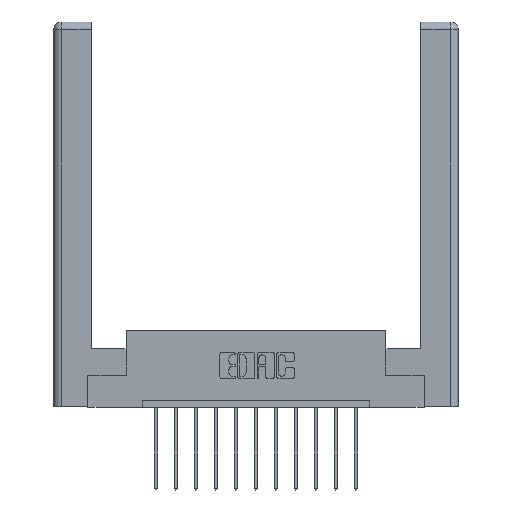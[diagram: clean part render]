
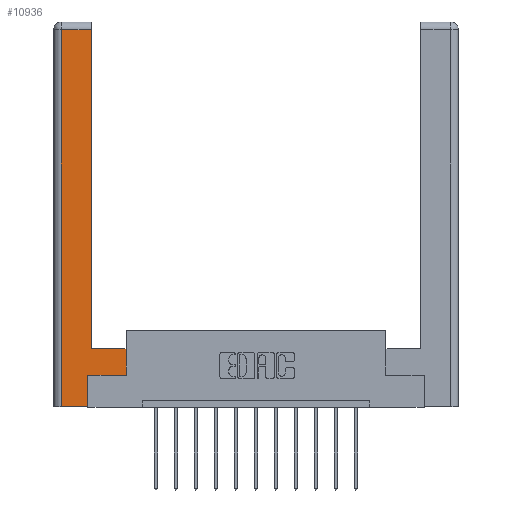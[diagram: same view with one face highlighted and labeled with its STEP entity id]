
A CAD part, top view. The second image highlights one B-rep face of the part: STEP entity #10936.
In plain terms, the highlighted planar face has unit normal (0, 0, 1).
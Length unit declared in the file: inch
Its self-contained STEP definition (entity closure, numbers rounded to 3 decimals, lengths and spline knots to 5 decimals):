
#6 = FACE_OUTER_BOUND ( 'NONE', #13969, .T. ) ;
#289 = DIRECTION ( 'NONE',  ( 1., 0., 0. ) ) ;
#618 = CARTESIAN_POINT ( 'NONE',  ( 0., 0., 0. ) ) ;
#725 = CARTESIAN_POINT ( 'NONE',  ( 0.265, 0.245, 0. ) ) ;
#1170 = DIRECTION ( 'NONE',  ( 0., -1., 0. ) ) ;
#1248 = CARTESIAN_POINT ( 'NONE',  ( 0.0615, 0., 0. ) ) ;
#1255 = CARTESIAN_POINT ( 'NONE',  ( 0.295, 0.45, 0. ) ) ;
#1560 = VERTEX_POINT ( 'NONE', #14340 ) ;
#1608 = VECTOR ( 'NONE', #5920, 39.37008 ) ;
#1727 = AXIS2_PLACEMENT_3D ( 'NONE', #618, #10803, #11953 ) ;
#1862 = VECTOR ( 'NONE', #9137, 39.37008 ) ;
#2088 = ORIENTED_EDGE ( 'NONE', *, *, #3706, .T. ) ;
#2593 = EDGE_CURVE ( 'NONE', #11267, #3794, #4272, .T. ) ;
#2612 = CARTESIAN_POINT ( 'NONE',  ( 0.0615, 2.94, 0. ) ) ;
#2642 = ORIENTED_EDGE ( 'NONE', *, *, #10837, .T. ) ;
#2666 = CARTESIAN_POINT ( 'NONE',  ( 0.565, 0.245, 0. ) ) ;
#3118 = EDGE_CURVE ( 'NONE', #8657, #7747, #12504, .T. ) ;
#3403 = DIRECTION ( 'NONE',  ( 1., 0., 0. ) ) ;
#3669 = CARTESIAN_POINT ( 'NONE',  ( 0.265, 0., 0. ) ) ;
#3706 = EDGE_CURVE ( 'NONE', #14690, #8657, #5572, .T. ) ;
#3729 = DIRECTION ( 'NONE',  ( -1., 0., 0. ) ) ;
#3794 = VERTEX_POINT ( 'NONE', #1248 ) ;
#4035 = VERTEX_POINT ( 'NONE', #725 ) ;
#4204 = ORIENTED_EDGE ( 'NONE', *, *, #6866, .T. ) ;
#4272 = LINE ( 'NONE', #12767, #13080 ) ;
#4994 = CARTESIAN_POINT ( 'NONE',  ( 0.565, 0.245, 0. ) ) ;
#5572 = LINE ( 'NONE', #10207, #1862 ) ;
#5729 = ORIENTED_EDGE ( 'NONE', *, *, #10715, .T. ) ;
#5920 = DIRECTION ( 'NONE',  ( -1., 0., 0. ) ) ;
#6079 = CARTESIAN_POINT ( 'NONE',  ( 0.265, 0.245, 0. ) ) ;
#6152 = VECTOR ( 'NONE', #3729, 39.37008 ) ;
#6703 = LINE ( 'NONE', #2612, #6152 ) ;
#6866 = EDGE_CURVE ( 'NONE', #1560, #11267, #6703, .T. ) ;
#6891 = CARTESIAN_POINT ( 'NONE',  ( 0.265, 0., 0. ) ) ;
#7130 = ORIENTED_EDGE ( 'NONE', *, *, #7593, .T. ) ;
#7469 = CARTESIAN_POINT ( 'NONE',  ( 0.565, 0.45, 0. ) ) ;
#7593 = EDGE_CURVE ( 'NONE', #13030, #4035, #9563, .T. ) ;
#7747 = VERTEX_POINT ( 'NONE', #14266 ) ;
#8492 = DIRECTION ( 'NONE',  ( 0., 1., 0. ) ) ;
#8657 = VERTEX_POINT ( 'NONE', #7469 ) ;
#9137 = DIRECTION ( 'NONE',  ( 0., 1., 0. ) ) ;
#9563 = LINE ( 'NONE', #6079, #9916 ) ;
#9916 = VECTOR ( 'NONE', #14119, 39.37008 ) ;
#10207 = CARTESIAN_POINT ( 'NONE',  ( 0.565, 0.45, 0. ) ) ;
#10219 = VECTOR ( 'NONE', #8492, 39.37008 ) ;
#10420 = ORIENTED_EDGE ( 'NONE', *, *, #3118, .T. ) ;
#10474 = ORIENTED_EDGE ( 'NONE', *, *, #2593, .T. ) ;
#10715 = EDGE_CURVE ( 'NONE', #3794, #13030, #11173, .T. ) ;
#10803 = DIRECTION ( 'NONE',  ( 0., 0., -1. ) ) ;
#10837 = EDGE_CURVE ( 'NONE', #4035, #14690, #14543, .T. ) ;
#10936 = ADVANCED_FACE ( 'NONE', ( #6 ), #10998, .F. ) ;
#10998 = PLANE ( 'NONE',  #1727 ) ;
#11173 = LINE ( 'NONE', #6891, #13856 ) ;
#11267 = VERTEX_POINT ( 'NONE', #12851 ) ;
#11953 = DIRECTION ( 'NONE',  ( -1., 0., 0. ) ) ;
#12184 = LINE ( 'NONE', #14328, #10219 ) ;
#12237 = ORIENTED_EDGE ( 'NONE', *, *, #12816, .T. ) ;
#12504 = LINE ( 'NONE', #1255, #1608 ) ;
#12767 = CARTESIAN_POINT ( 'NONE',  ( 0.0615, 0., 0. ) ) ;
#12816 = EDGE_CURVE ( 'NONE', #7747, #1560, #12184, .T. ) ;
#12851 = CARTESIAN_POINT ( 'NONE',  ( 0.0615, 2.94, 0. ) ) ;
#13030 = VERTEX_POINT ( 'NONE', #3669 ) ;
#13080 = VECTOR ( 'NONE', #1170, 39.37008 ) ;
#13839 = VECTOR ( 'NONE', #289, 39.37008 ) ;
#13856 = VECTOR ( 'NONE', #3403, 39.37008 ) ;
#13969 = EDGE_LOOP ( 'NONE', ( #12237, #4204, #10474, #5729, #7130, #2642, #2088, #10420 ) ) ;
#14119 = DIRECTION ( 'NONE',  ( 0., 1., 0. ) ) ;
#14266 = CARTESIAN_POINT ( 'NONE',  ( 0.295, 0.45, 0. ) ) ;
#14328 = CARTESIAN_POINT ( 'NONE',  ( 0.295, 3., 0. ) ) ;
#14340 = CARTESIAN_POINT ( 'NONE',  ( 0.295, 2.94, 0. ) ) ;
#14543 = LINE ( 'NONE', #4994, #13839 ) ;
#14690 = VERTEX_POINT ( 'NONE', #2666 ) ;
